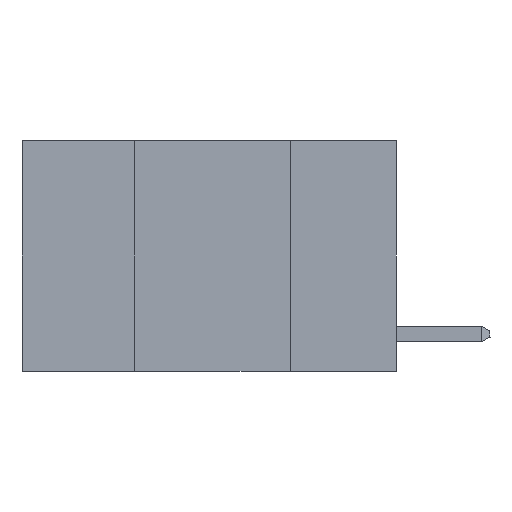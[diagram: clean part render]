
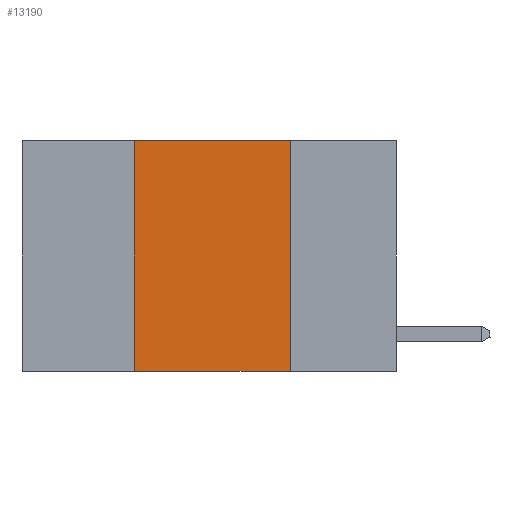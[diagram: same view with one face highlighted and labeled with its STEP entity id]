
A CAD part, left-side view. The second image highlights one B-rep face of the part: STEP entity #13190.
In plain terms, the highlighted planar face has unit normal (-1, 0, 0).
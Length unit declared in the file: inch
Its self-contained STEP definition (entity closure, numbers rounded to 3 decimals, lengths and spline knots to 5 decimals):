
#100 = CARTESIAN_POINT ( 'NONE',  ( 0., 0.17, 0. ) ) ;
#310 = VECTOR ( 'NONE', #7934, 39.37008 ) ;
#872 = EDGE_CURVE ( 'NONE', #11530, #13123, #7689, .T. ) ;
#1975 = ORIENTED_EDGE ( 'NONE', *, *, #872, .F. ) ;
#1980 = LINE ( 'NONE', #4488, #310 ) ;
#2196 = EDGE_CURVE ( 'NONE', #15238, #13123, #1980, .T. ) ;
#2202 = PLANE ( 'NONE',  #11742 ) ;
#2577 = EDGE_CURVE ( 'NONE', #15238, #12886, #3863, .T. ) ;
#2785 = ORIENTED_EDGE ( 'NONE', *, *, #2577, .F. ) ;
#3084 = CARTESIAN_POINT ( 'NONE',  ( 0., 0.17, 0. ) ) ;
#3223 = CARTESIAN_POINT ( 'NONE',  ( 0., 0.17, -0.37 ) ) ;
#3863 = LINE ( 'NONE', #9952, #8573 ) ;
#4488 = CARTESIAN_POINT ( 'NONE',  ( 0., 0.6, -0.37 ) ) ;
#4846 = DIRECTION ( 'NONE',  ( 0., 0., -1. ) ) ;
#5430 = EDGE_CURVE ( 'NONE', #12886, #11530, #7932, .T. ) ;
#6292 = DIRECTION ( 'NONE',  ( 0., 0., -1. ) ) ;
#7127 = FACE_OUTER_BOUND ( 'NONE', #11700, .T. ) ;
#7689 = LINE ( 'NONE', #3084, #14951 ) ;
#7932 = LINE ( 'NONE', #9407, #8992 ) ;
#7934 = DIRECTION ( 'NONE',  ( 0., -1., 0. ) ) ;
#8573 = VECTOR ( 'NONE', #14730, 39.37008 ) ;
#8992 = VECTOR ( 'NONE', #12961, 39.37008 ) ;
#9232 = ORIENTED_EDGE ( 'NONE', *, *, #2196, .T. ) ;
#9407 = CARTESIAN_POINT ( 'NONE',  ( 0., 0.6, 0. ) ) ;
#9542 = DIRECTION ( 'NONE',  ( 1., 0., 0. ) ) ;
#9632 = ORIENTED_EDGE ( 'NONE', *, *, #5430, .F. ) ;
#9952 = CARTESIAN_POINT ( 'NONE',  ( 0., 0.42, 0. ) ) ;
#11530 = VERTEX_POINT ( 'NONE', #100 ) ;
#11700 = EDGE_LOOP ( 'NONE', ( #1975, #9632, #2785, #9232 ) ) ;
#11742 = AXIS2_PLACEMENT_3D ( 'NONE', #14324, #9542, #4846 ) ;
#12242 = CARTESIAN_POINT ( 'NONE',  ( 0., 0.42, 0. ) ) ;
#12886 = VERTEX_POINT ( 'NONE', #12242 ) ;
#12961 = DIRECTION ( 'NONE',  ( 0., -1., 0. ) ) ;
#13123 = VERTEX_POINT ( 'NONE', #3223 ) ;
#13163 = CARTESIAN_POINT ( 'NONE',  ( 0., 0.42, -0.37 ) ) ;
#13190 = ADVANCED_FACE ( 'NONE', ( #7127 ), #2202, .F. ) ;
#14324 = CARTESIAN_POINT ( 'NONE',  ( 0., 0.6, 0. ) ) ;
#14730 = DIRECTION ( 'NONE',  ( 0., 0., 1. ) ) ;
#14951 = VECTOR ( 'NONE', #6292, 39.37008 ) ;
#15238 = VERTEX_POINT ( 'NONE', #13163 ) ;
